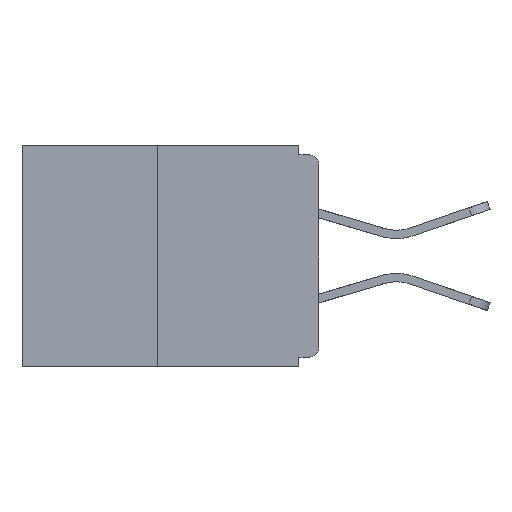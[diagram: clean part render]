
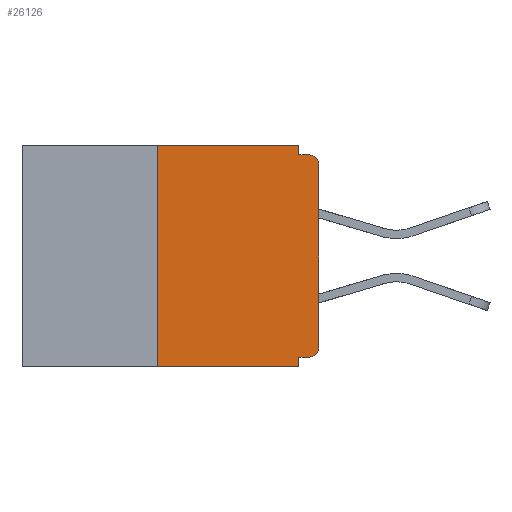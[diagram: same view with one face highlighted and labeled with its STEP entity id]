
A CAD part, left-side view. The second image highlights one B-rep face of the part: STEP entity #26126.
In plain terms, the highlighted planar face has unit normal (-1, 0, 0).
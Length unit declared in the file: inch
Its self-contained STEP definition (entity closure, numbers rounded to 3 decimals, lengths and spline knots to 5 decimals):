
#419 = VECTOR ( 'NONE', #6137, 39.37008 ) ;
#548 = EDGE_CURVE ( 'NONE', #7192, #23960, #5974, .T. ) ;
#616 = VERTEX_POINT ( 'NONE', #24414 ) ;
#700 = AXIS2_PLACEMENT_3D ( 'NONE', #23091, #9528, #14085 ) ;
#1301 = EDGE_CURVE ( 'NONE', #11868, #20804, #13376, .T. ) ;
#2214 = ORIENTED_EDGE ( 'NONE', *, *, #15319, .F. ) ;
#2347 = ORIENTED_EDGE ( 'NONE', *, *, #1301, .T. ) ;
#2927 = CARTESIAN_POINT ( 'NONE',  ( 0., 0., -0.313 ) ) ;
#3866 = CARTESIAN_POINT ( 'NONE',  ( 0., 0., -0.015 ) ) ;
#3961 = DIRECTION ( 'NONE',  ( 0., -1., 0. ) ) ;
#4045 = CARTESIAN_POINT ( 'NONE',  ( 0., 0., 0. ) ) ;
#4614 = CARTESIAN_POINT ( 'NONE',  ( 0., 0.25, 0. ) ) ;
#4956 = DIRECTION ( 'NONE',  ( 0., 0., -1. ) ) ;
#5237 = VECTOR ( 'NONE', #13313, 39.37008 ) ;
#5568 = LINE ( 'NONE', #25273, #18679 ) ;
#5902 = VECTOR ( 'NONE', #21928, 39.37008 ) ;
#5974 = LINE ( 'NONE', #4045, #5237 ) ;
#6137 = DIRECTION ( 'NONE',  ( 0., 0., 1. ) ) ;
#6604 = CARTESIAN_POINT ( 'NONE',  ( 0., 0.031, -0.328 ) ) ;
#7192 = VERTEX_POINT ( 'NONE', #2927 ) ;
#7563 = DIRECTION ( 'NONE',  ( 0., 1., 0. ) ) ;
#7873 = DIRECTION ( 'NONE',  ( 0., 0., -1. ) ) ;
#8073 = CARTESIAN_POINT ( 'NONE',  ( 0., 0.46, -0.343 ) ) ;
#8279 = CARTESIAN_POINT ( 'NONE',  ( 0., 0.46, 0. ) ) ;
#8473 = VECTOR ( 'NONE', #7563, 39.37008 ) ;
#8696 = VECTOR ( 'NONE', #7873, 39.37008 ) ;
#9528 = DIRECTION ( 'NONE',  ( -1., 0., 0. ) ) ;
#9607 = DIRECTION ( 'NONE',  ( 1., 0., 0. ) ) ;
#10231 = EDGE_CURVE ( 'NONE', #616, #25623, #15082, .T. ) ;
#10366 = ORIENTED_EDGE ( 'NONE', *, *, #14923, .T. ) ;
#11402 = CARTESIAN_POINT ( 'NONE',  ( 0., 0.015, -0.03 ) ) ;
#11868 = VERTEX_POINT ( 'NONE', #28287 ) ;
#11964 = CARTESIAN_POINT ( 'NONE',  ( 0., 0.46, 0. ) ) ;
#13313 = DIRECTION ( 'NONE',  ( 0., 0., 1. ) ) ;
#13376 = LINE ( 'NONE', #8073, #26486 ) ;
#13698 = DIRECTION ( 'NONE',  ( -1., 0., 0. ) ) ;
#14085 = DIRECTION ( 'NONE',  ( 0., 0., -1. ) ) ;
#14716 = DIRECTION ( 'NONE',  ( 0., -1., 0. ) ) ;
#14923 = EDGE_CURVE ( 'NONE', #23960, #25623, #23753, .T. ) ;
#15082 = LINE ( 'NONE', #3866, #15804 ) ;
#15319 = EDGE_CURVE ( 'NONE', #11868, #26862, #16677, .T. ) ;
#15464 = LINE ( 'NONE', #8279, #5902 ) ;
#15644 = ORIENTED_EDGE ( 'NONE', *, *, #20439, .F. ) ;
#15715 = FACE_OUTER_BOUND ( 'NONE', #23331, .T. ) ;
#15804 = VECTOR ( 'NONE', #3961, 39.37008 ) ;
#15984 = DIRECTION ( 'NONE',  ( 0., 0., -1. ) ) ;
#16330 = CARTESIAN_POINT ( 'NONE',  ( 0., 0.015, -0.015 ) ) ;
#16541 = PLANE ( 'NONE',  #18726 ) ;
#16612 = ORIENTED_EDGE ( 'NONE', *, *, #18079, .F. ) ;
#16677 = LINE ( 'NONE', #28563, #419 ) ;
#17408 = ORIENTED_EDGE ( 'NONE', *, *, #23686, .F. ) ;
#17631 = CIRCLE ( 'NONE', #700, 0.015 ) ;
#17974 = ORIENTED_EDGE ( 'NONE', *, *, #548, .T. ) ;
#18079 = EDGE_CURVE ( 'NONE', #23165, #25232, #27939, .T. ) ;
#18679 = VECTOR ( 'NONE', #21174, 39.37008 ) ;
#18726 = AXIS2_PLACEMENT_3D ( 'NONE', #11964, #9607, #4956 ) ;
#18836 = ORIENTED_EDGE ( 'NONE', *, *, #10231, .F. ) ;
#19072 = AXIS2_PLACEMENT_3D ( 'NONE', #11402, #13698, #15984 ) ;
#19991 = CARTESIAN_POINT ( 'NONE',  ( 0., 0., -0.03 ) ) ;
#20439 = EDGE_CURVE ( 'NONE', #26862, #26041, #15464, .T. ) ;
#20668 = EDGE_CURVE ( 'NONE', #26041, #616, #23933, .T. ) ;
#20804 = VERTEX_POINT ( 'NONE', #27130 ) ;
#20885 = CARTESIAN_POINT ( 'NONE',  ( 0., 0., -0.328 ) ) ;
#21174 = DIRECTION ( 'NONE',  ( 0., 0., -1. ) ) ;
#21928 = DIRECTION ( 'NONE',  ( 0., -1., 0. ) ) ;
#23091 = CARTESIAN_POINT ( 'NONE',  ( 0., 0.015, -0.313 ) ) ;
#23165 = VERTEX_POINT ( 'NONE', #26625 ) ;
#23331 = EDGE_LOOP ( 'NONE', ( #15644, #2214, #2347, #17408, #16612, #23820, #17974, #10366, #18836, #27842 ) ) ;
#23528 = EDGE_CURVE ( 'NONE', #23165, #7192, #17631, .T. ) ;
#23686 = EDGE_CURVE ( 'NONE', #25232, #20804, #5568, .T. ) ;
#23753 = CIRCLE ( 'NONE', #19072, 0.015 ) ;
#23820 = ORIENTED_EDGE ( 'NONE', *, *, #23528, .T. ) ;
#23933 = LINE ( 'NONE', #26178, #8696 ) ;
#23960 = VERTEX_POINT ( 'NONE', #19991 ) ;
#24414 = CARTESIAN_POINT ( 'NONE',  ( 0., 0.031, -0.015 ) ) ;
#25232 = VERTEX_POINT ( 'NONE', #6604 ) ;
#25273 = CARTESIAN_POINT ( 'NONE',  ( 0., 0.031, -0.343 ) ) ;
#25623 = VERTEX_POINT ( 'NONE', #16330 ) ;
#25893 = CARTESIAN_POINT ( 'NONE',  ( 0., 0.031, 0. ) ) ;
#26041 = VERTEX_POINT ( 'NONE', #25893 ) ;
#26126 = ADVANCED_FACE ( 'NONE', ( #15715 ), #16541, .F. ) ;
#26178 = CARTESIAN_POINT ( 'NONE',  ( 0., 0.031, 0. ) ) ;
#26486 = VECTOR ( 'NONE', #14716, 39.37008 ) ;
#26625 = CARTESIAN_POINT ( 'NONE',  ( 0., 0.015, -0.328 ) ) ;
#26862 = VERTEX_POINT ( 'NONE', #4614 ) ;
#27130 = CARTESIAN_POINT ( 'NONE',  ( 0., 0.031, -0.343 ) ) ;
#27842 = ORIENTED_EDGE ( 'NONE', *, *, #20668, .F. ) ;
#27939 = LINE ( 'NONE', #20885, #8473 ) ;
#28287 = CARTESIAN_POINT ( 'NONE',  ( 0., 0.25, -0.343 ) ) ;
#28563 = CARTESIAN_POINT ( 'NONE',  ( 0., 0.25, 0. ) ) ;
